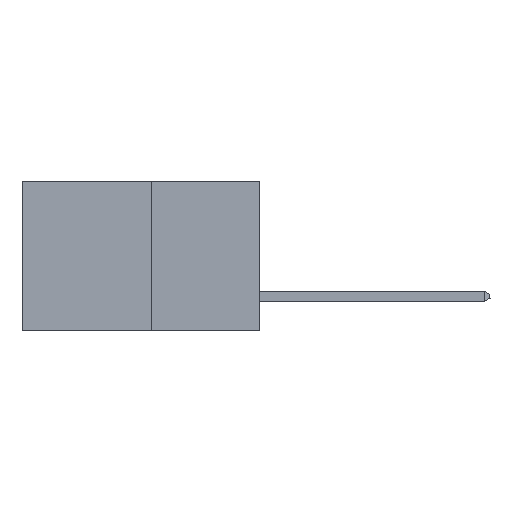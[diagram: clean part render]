
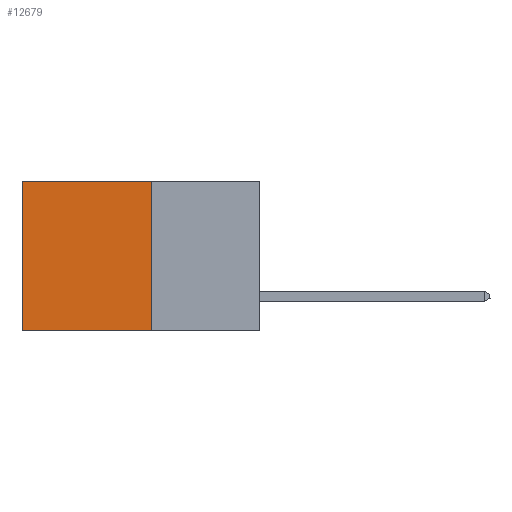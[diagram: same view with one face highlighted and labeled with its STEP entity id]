
A CAD part, left-side view. The second image highlights one B-rep face of the part: STEP entity #12679.
In plain terms, the highlighted planar face has unit normal (-1, 0, 0).
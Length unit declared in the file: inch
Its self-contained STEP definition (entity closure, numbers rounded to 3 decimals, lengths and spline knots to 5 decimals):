
#577 = VERTEX_POINT ( 'NONE', #7159 ) ;
#582 = DIRECTION ( 'NONE',  ( 1., 0., 0. ) ) ;
#1571 = ORIENTED_EDGE ( 'NONE', *, *, #10910, .F. ) ;
#1830 = CARTESIAN_POINT ( 'NONE',  ( 0.277, 0.27, 0. ) ) ;
#1951 = PLANE ( 'NONE',  #3967 ) ;
#2141 = CARTESIAN_POINT ( 'NONE',  ( 0.277, 0.27, -0.37 ) ) ;
#2611 = DIRECTION ( 'NONE',  ( 0., 1., 0. ) ) ;
#2790 = CARTESIAN_POINT ( 'NONE',  ( 0.277, 0.59, -0.37 ) ) ;
#3027 = VECTOR ( 'NONE', #5235, 39.37008 ) ;
#3292 = LINE ( 'NONE', #4357, #9445 ) ;
#3446 = EDGE_LOOP ( 'NONE', ( #15601, #1571, #12780, #9551 ) ) ;
#3967 = AXIS2_PLACEMENT_3D ( 'NONE', #17303, #582, #10431 ) ;
#4357 = CARTESIAN_POINT ( 'NONE',  ( 0.277, 0.27, -0.37 ) ) ;
#5235 = DIRECTION ( 'NONE',  ( 0., 0., -1. ) ) ;
#5500 = CARTESIAN_POINT ( 'NONE',  ( 0.277, 0.27, 0. ) ) ;
#5804 = VERTEX_POINT ( 'NONE', #9695 ) ;
#5920 = LINE ( 'NONE', #2141, #16525 ) ;
#6186 = FACE_OUTER_BOUND ( 'NONE', #3446, .T. ) ;
#7159 = CARTESIAN_POINT ( 'NONE',  ( 0.277, 0.59, 0. ) ) ;
#9445 = VECTOR ( 'NONE', #11259, 39.37008 ) ;
#9551 = ORIENTED_EDGE ( 'NONE', *, *, #10480, .T. ) ;
#9695 = CARTESIAN_POINT ( 'NONE',  ( 0.277, 0.27, -0.37 ) ) ;
#9827 = VECTOR ( 'NONE', #2611, 39.37008 ) ;
#10431 = DIRECTION ( 'NONE',  ( 0., 0., -1. ) ) ;
#10480 = EDGE_CURVE ( 'NONE', #10766, #577, #12628, .T. ) ;
#10766 = VERTEX_POINT ( 'NONE', #1830 ) ;
#10910 = EDGE_CURVE ( 'NONE', #5804, #16141, #5920, .T. ) ;
#11259 = DIRECTION ( 'NONE',  ( 0., 0., -1. ) ) ;
#12144 = CARTESIAN_POINT ( 'NONE',  ( 0.277, 0.59, -0.37 ) ) ;
#12628 = LINE ( 'NONE', #5500, #9827 ) ;
#12679 = ADVANCED_FACE ( 'NONE', ( #6186 ), #1951, .F. ) ;
#12780 = ORIENTED_EDGE ( 'NONE', *, *, #15564, .F. ) ;
#13372 = DIRECTION ( 'NONE',  ( 0., 1., 0. ) ) ;
#14158 = EDGE_CURVE ( 'NONE', #577, #16141, #17803, .T. ) ;
#15564 = EDGE_CURVE ( 'NONE', #10766, #5804, #3292, .T. ) ;
#15601 = ORIENTED_EDGE ( 'NONE', *, *, #14158, .T. ) ;
#16141 = VERTEX_POINT ( 'NONE', #2790 ) ;
#16525 = VECTOR ( 'NONE', #13372, 39.37008 ) ;
#17303 = CARTESIAN_POINT ( 'NONE',  ( 0.277, 0.27, -0.37 ) ) ;
#17803 = LINE ( 'NONE', #12144, #3027 ) ;
